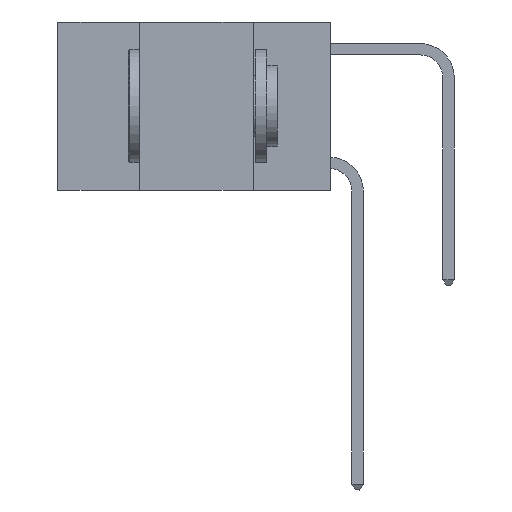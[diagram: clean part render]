
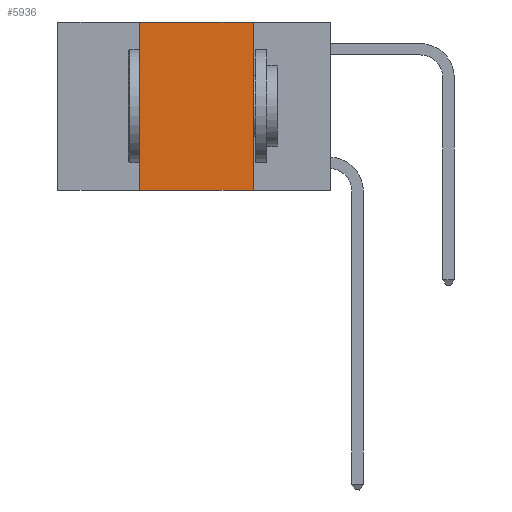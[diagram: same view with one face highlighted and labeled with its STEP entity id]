
A CAD part, left-side view. The second image highlights one B-rep face of the part: STEP entity #5936.
In plain terms, the highlighted planar face has unit normal (-1, 0, 0).
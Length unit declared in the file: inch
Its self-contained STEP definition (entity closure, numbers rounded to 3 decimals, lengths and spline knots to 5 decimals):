
#421 = CARTESIAN_POINT ( 'NONE',  ( 0., 0.6, -0.37 ) ) ;
#452 = DIRECTION ( 'NONE',  ( 0., -1., 0. ) ) ;
#1090 = EDGE_CURVE ( 'NONE', #1882, #10433, #11685, .T. ) ;
#1109 = DIRECTION ( 'NONE',  ( 0., 0., -1. ) ) ;
#1173 = VERTEX_POINT ( 'NONE', #13843 ) ;
#1882 = VERTEX_POINT ( 'NONE', #13428 ) ;
#2677 = VECTOR ( 'NONE', #452, 39.37008 ) ;
#3283 = VECTOR ( 'NONE', #9746, 39.37008 ) ;
#3442 = LINE ( 'NONE', #7247, #17907 ) ;
#3839 = LINE ( 'NONE', #20856, #3283 ) ;
#4939 = EDGE_CURVE ( 'NONE', #1882, #10871, #3839, .T. ) ;
#5052 = CARTESIAN_POINT ( 'NONE',  ( 0., 0.6, 0. ) ) ;
#5936 = ADVANCED_FACE ( 'NONE', ( #15981 ), #10725, .F. ) ;
#6807 = CARTESIAN_POINT ( 'NONE',  ( 0., 0.6, 0. ) ) ;
#7247 = CARTESIAN_POINT ( 'NONE',  ( 0., 0.17, 0. ) ) ;
#7508 = EDGE_CURVE ( 'NONE', #1173, #10433, #3442, .T. ) ;
#8866 = DIRECTION ( 'NONE',  ( 0., -1., 0. ) ) ;
#8872 = EDGE_CURVE ( 'NONE', #10871, #1173, #20723, .T. ) ;
#9746 = DIRECTION ( 'NONE',  ( 0., 0., 1. ) ) ;
#10433 = VERTEX_POINT ( 'NONE', #22652 ) ;
#10725 = PLANE ( 'NONE',  #19041 ) ;
#10871 = VERTEX_POINT ( 'NONE', #23825 ) ;
#11514 = EDGE_LOOP ( 'NONE', ( #20196, #11755, #22678, #17831 ) ) ;
#11685 = LINE ( 'NONE', #421, #2677 ) ;
#11755 = ORIENTED_EDGE ( 'NONE', *, *, #8872, .F. ) ;
#12601 = DIRECTION ( 'NONE',  ( 1., 0., 0. ) ) ;
#13428 = CARTESIAN_POINT ( 'NONE',  ( 0., 0.42, -0.37 ) ) ;
#13843 = CARTESIAN_POINT ( 'NONE',  ( 0., 0.17, 0. ) ) ;
#14707 = VECTOR ( 'NONE', #8866, 39.37008 ) ;
#15981 = FACE_OUTER_BOUND ( 'NONE', #11514, .T. ) ;
#17831 = ORIENTED_EDGE ( 'NONE', *, *, #1090, .T. ) ;
#17907 = VECTOR ( 'NONE', #22174, 39.37008 ) ;
#19041 = AXIS2_PLACEMENT_3D ( 'NONE', #6807, #12601, #1109 ) ;
#20196 = ORIENTED_EDGE ( 'NONE', *, *, #7508, .F. ) ;
#20723 = LINE ( 'NONE', #5052, #14707 ) ;
#20856 = CARTESIAN_POINT ( 'NONE',  ( 0., 0.42, 0. ) ) ;
#22174 = DIRECTION ( 'NONE',  ( 0., 0., -1. ) ) ;
#22652 = CARTESIAN_POINT ( 'NONE',  ( 0., 0.17, -0.37 ) ) ;
#22678 = ORIENTED_EDGE ( 'NONE', *, *, #4939, .F. ) ;
#23825 = CARTESIAN_POINT ( 'NONE',  ( 0., 0.42, 0. ) ) ;
